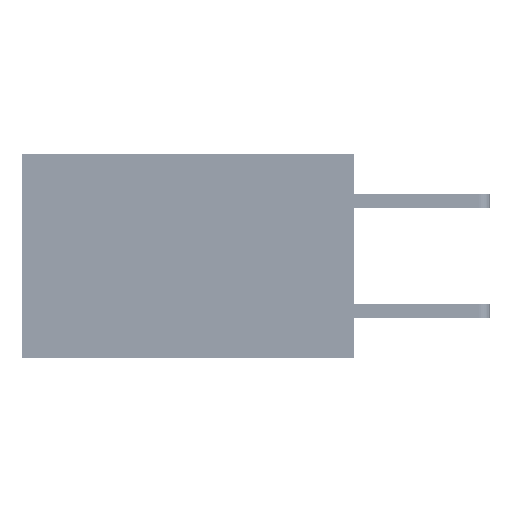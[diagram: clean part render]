
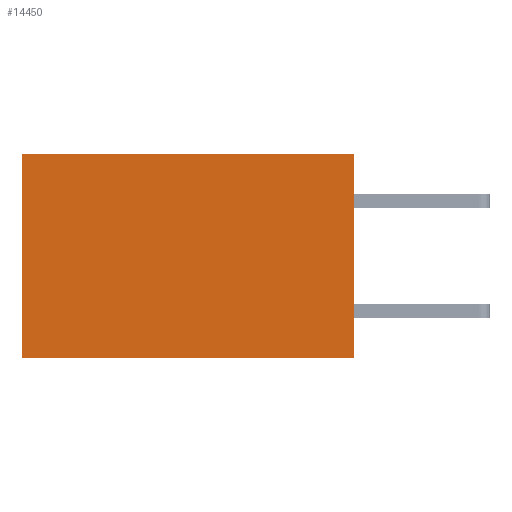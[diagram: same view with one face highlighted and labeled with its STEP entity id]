
A CAD part, left-side view. The second image highlights one B-rep face of the part: STEP entity #14450.
In plain terms, the highlighted planar face has unit normal (-1, 0, 0).
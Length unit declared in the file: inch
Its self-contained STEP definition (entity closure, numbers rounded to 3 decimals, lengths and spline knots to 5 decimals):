
#223 = LINE ( 'NONE', #8104, #5987 ) ;
#2899 = AXIS2_PLACEMENT_3D ( 'NONE', #41424, #23424, #16362 ) ;
#5987 = VECTOR ( 'NONE', #43562, 39.37008 ) ;
#6514 = VERTEX_POINT ( 'NONE', #31547 ) ;
#8104 = CARTESIAN_POINT ( 'NONE',  ( 0.2875, 0.6, 0. ) ) ;
#8346 = CARTESIAN_POINT ( 'NONE',  ( 0.2875, 0., -0.37 ) ) ;
#9888 = DIRECTION ( 'NONE',  ( 0., 0., -1. ) ) ;
#10002 = ORIENTED_EDGE ( 'NONE', *, *, #15408, .T. ) ;
#11423 = EDGE_CURVE ( 'NONE', #43086, #6514, #13887, .T. ) ;
#11935 = FACE_OUTER_BOUND ( 'NONE', #22942, .T. ) ;
#12026 = PLANE ( 'NONE',  #2899 ) ;
#13887 = LINE ( 'NONE', #42975, #43204 ) ;
#14014 = CARTESIAN_POINT ( 'NONE',  ( 0.2875, 0., 0. ) ) ;
#14450 = ADVANCED_FACE ( 'NONE', ( #11935 ), #12026, .F. ) ;
#15408 = EDGE_CURVE ( 'NONE', #43086, #43545, #18733, .T. ) ;
#16174 = EDGE_CURVE ( 'NONE', #43545, #26737, #223, .T. ) ;
#16362 = DIRECTION ( 'NONE',  ( 0., 0., -1. ) ) ;
#17187 = ORIENTED_EDGE ( 'NONE', *, *, #45025, .F. ) ;
#17577 = VECTOR ( 'NONE', #17895, 39.37008 ) ;
#17895 = DIRECTION ( 'NONE',  ( 0., 1., 0. ) ) ;
#18239 = ORIENTED_EDGE ( 'NONE', *, *, #11423, .F. ) ;
#18733 = LINE ( 'NONE', #14014, #17577 ) ;
#20949 = LINE ( 'NONE', #8346, #43966 ) ;
#22942 = EDGE_LOOP ( 'NONE', ( #31299, #17187, #18239, #10002 ) ) ;
#23424 = DIRECTION ( 'NONE',  ( 1., 0., 0. ) ) ;
#25669 = CARTESIAN_POINT ( 'NONE',  ( 0.2875, 0.6, 0. ) ) ;
#26664 = CARTESIAN_POINT ( 'NONE',  ( 0.2875, 0., 0. ) ) ;
#26737 = VERTEX_POINT ( 'NONE', #31508 ) ;
#31299 = ORIENTED_EDGE ( 'NONE', *, *, #16174, .T. ) ;
#31508 = CARTESIAN_POINT ( 'NONE',  ( 0.2875, 0.6, -0.37 ) ) ;
#31547 = CARTESIAN_POINT ( 'NONE',  ( 0.2875, 0., -0.37 ) ) ;
#40907 = DIRECTION ( 'NONE',  ( 0., 1., 0. ) ) ;
#41424 = CARTESIAN_POINT ( 'NONE',  ( 0.2875, 0., 0. ) ) ;
#42975 = CARTESIAN_POINT ( 'NONE',  ( 0.2875, 0., 0. ) ) ;
#43086 = VERTEX_POINT ( 'NONE', #26664 ) ;
#43204 = VECTOR ( 'NONE', #9888, 39.37008 ) ;
#43545 = VERTEX_POINT ( 'NONE', #25669 ) ;
#43562 = DIRECTION ( 'NONE',  ( 0., 0., -1. ) ) ;
#43966 = VECTOR ( 'NONE', #40907, 39.37008 ) ;
#45025 = EDGE_CURVE ( 'NONE', #6514, #26737, #20949, .T. ) ;
